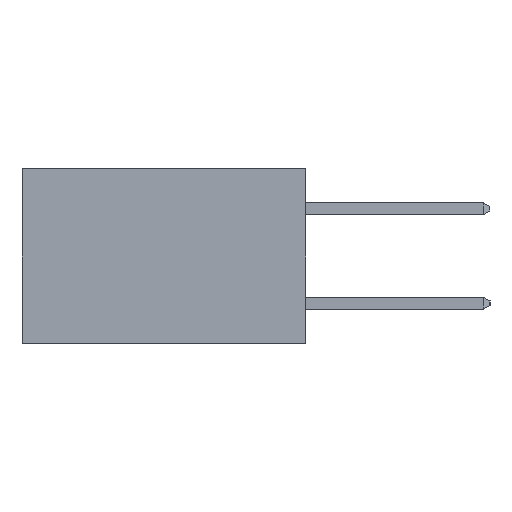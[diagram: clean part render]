
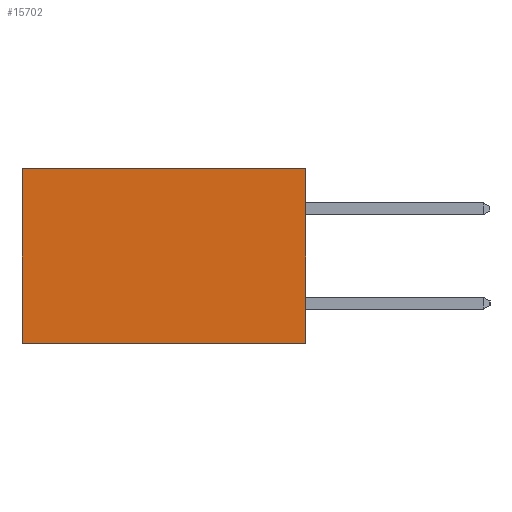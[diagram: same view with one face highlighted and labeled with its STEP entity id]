
A CAD part, left-side view. The second image highlights one B-rep face of the part: STEP entity #15702.
In plain terms, the highlighted planar face has unit normal (-1, 0, 0).
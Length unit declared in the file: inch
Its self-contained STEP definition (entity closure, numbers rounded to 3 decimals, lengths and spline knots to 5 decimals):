
#313 = LINE ( 'NONE', #18890, #17151 ) ;
#661 = EDGE_CURVE ( 'NONE', #6761, #12344, #21042, .T. ) ;
#932 = EDGE_CURVE ( 'NONE', #12344, #1799, #2987, .T. ) ;
#945 = VERTEX_POINT ( 'NONE', #12735 ) ;
#1093 = EDGE_CURVE ( 'NONE', #6761, #945, #313, .T. ) ;
#1145 = ORIENTED_EDGE ( 'NONE', *, *, #661, .F. ) ;
#1323 = CARTESIAN_POINT ( 'NONE',  ( 0.2615, 0., 0. ) ) ;
#1609 = EDGE_CURVE ( 'NONE', #945, #1799, #3933, .T. ) ;
#1799 = VERTEX_POINT ( 'NONE', #17880 ) ;
#2327 = ORIENTED_EDGE ( 'NONE', *, *, #1093, .T. ) ;
#2987 = LINE ( 'NONE', #10928, #20254 ) ;
#3772 = CARTESIAN_POINT ( 'NONE',  ( 0.2615, 0.6, -0.37 ) ) ;
#3933 = LINE ( 'NONE', #3772, #8429 ) ;
#4767 = PLANE ( 'NONE',  #19483 ) ;
#4839 = DIRECTION ( 'NONE',  ( 1., 0., 0. ) ) ;
#4882 = FACE_OUTER_BOUND ( 'NONE', #16921, .T. ) ;
#6761 = VERTEX_POINT ( 'NONE', #1323 ) ;
#8429 = VECTOR ( 'NONE', #12392, 39.37008 ) ;
#9726 = ORIENTED_EDGE ( 'NONE', *, *, #1609, .T. ) ;
#10928 = CARTESIAN_POINT ( 'NONE',  ( 0.2615, 0., -0.37 ) ) ;
#11948 = CARTESIAN_POINT ( 'NONE',  ( 0.2615, 0., -0.37 ) ) ;
#12344 = VERTEX_POINT ( 'NONE', #13328 ) ;
#12392 = DIRECTION ( 'NONE',  ( 0., 0., -1. ) ) ;
#12394 = DIRECTION ( 'NONE',  ( 0., 0., -1. ) ) ;
#12735 = CARTESIAN_POINT ( 'NONE',  ( 0.2615, 0.6, 0. ) ) ;
#13328 = CARTESIAN_POINT ( 'NONE',  ( 0.2615, 0., -0.37 ) ) ;
#14927 = CARTESIAN_POINT ( 'NONE',  ( 0.2615, 0., -0.37 ) ) ;
#15702 = ADVANCED_FACE ( 'NONE', ( #4882 ), #4767, .F. ) ;
#16586 = DIRECTION ( 'NONE',  ( 0., 0., -1. ) ) ;
#16674 = VECTOR ( 'NONE', #12394, 39.37008 ) ;
#16921 = EDGE_LOOP ( 'NONE', ( #9726, #18985, #1145, #2327 ) ) ;
#17151 = VECTOR ( 'NONE', #21272, 39.37008 ) ;
#17880 = CARTESIAN_POINT ( 'NONE',  ( 0.2615, 0.6, -0.37 ) ) ;
#18610 = DIRECTION ( 'NONE',  ( 0., 1., 0. ) ) ;
#18890 = CARTESIAN_POINT ( 'NONE',  ( 0.2615, 0., 0. ) ) ;
#18985 = ORIENTED_EDGE ( 'NONE', *, *, #932, .F. ) ;
#19483 = AXIS2_PLACEMENT_3D ( 'NONE', #14927, #4839, #16586 ) ;
#20254 = VECTOR ( 'NONE', #18610, 39.37008 ) ;
#21042 = LINE ( 'NONE', #11948, #16674 ) ;
#21272 = DIRECTION ( 'NONE',  ( 0., 1., 0. ) ) ;
